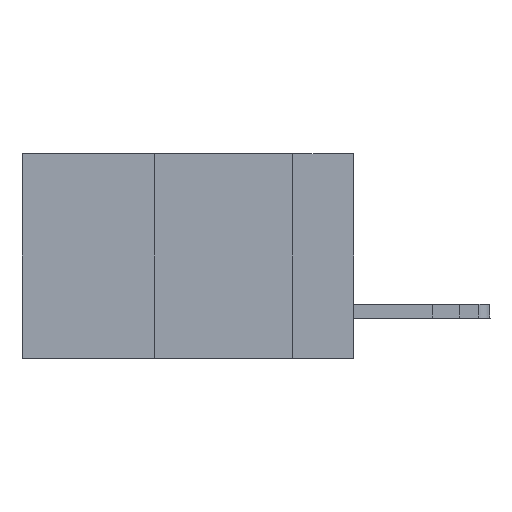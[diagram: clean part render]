
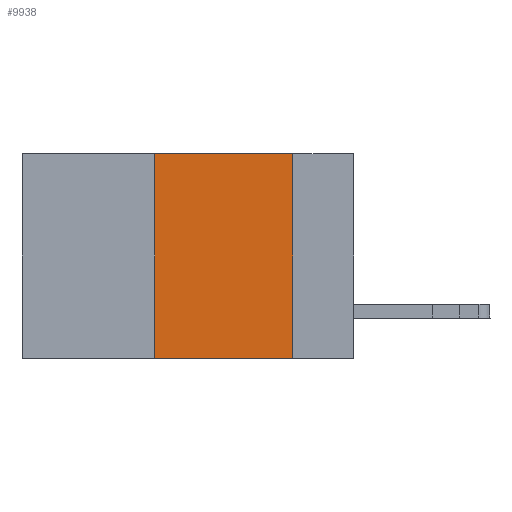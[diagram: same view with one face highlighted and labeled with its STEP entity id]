
A CAD part, left-side view. The second image highlights one B-rep face of the part: STEP entity #9938.
In plain terms, the highlighted planar face has unit normal (-1, 0, 0).
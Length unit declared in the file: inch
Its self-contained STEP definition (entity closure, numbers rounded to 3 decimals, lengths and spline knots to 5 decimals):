
#1124 = VERTEX_POINT ( 'NONE', #6725 ) ;
#1776 = LINE ( 'NONE', #12048, #10622 ) ;
#1821 = DIRECTION ( 'NONE',  ( 0., -1., 0. ) ) ;
#2107 = CARTESIAN_POINT ( 'NONE',  ( 0., 0.11, 0. ) ) ;
#3855 = CARTESIAN_POINT ( 'NONE',  ( 0., 0.11, 0. ) ) ;
#4981 = EDGE_CURVE ( 'NONE', #1124, #7231, #6101, .T. ) ;
#5998 = EDGE_CURVE ( 'NONE', #9878, #8299, #15876, .T. ) ;
#6101 = LINE ( 'NONE', #16797, #10992 ) ;
#6137 = CARTESIAN_POINT ( 'NONE',  ( 0., 0.36, 0. ) ) ;
#6437 = ORIENTED_EDGE ( 'NONE', *, *, #5998, .F. ) ;
#6725 = CARTESIAN_POINT ( 'NONE',  ( 0., 0.36, -0.37 ) ) ;
#7231 = VERTEX_POINT ( 'NONE', #14925 ) ;
#7925 = VECTOR ( 'NONE', #18541, 39.37008 ) ;
#8299 = VERTEX_POINT ( 'NONE', #3855 ) ;
#8394 = PLANE ( 'NONE',  #9184 ) ;
#8455 = DIRECTION ( 'NONE',  ( 0., 0., -1. ) ) ;
#9184 = AXIS2_PLACEMENT_3D ( 'NONE', #11413, #17451, #8455 ) ;
#9392 = ORIENTED_EDGE ( 'NONE', *, *, #9624, .F. ) ;
#9624 = EDGE_CURVE ( 'NONE', #1124, #9878, #1776, .T. ) ;
#9645 = CARTESIAN_POINT ( 'NONE',  ( 0., 0.6, 0. ) ) ;
#9878 = VERTEX_POINT ( 'NONE', #6137 ) ;
#9938 = ADVANCED_FACE ( 'NONE', ( #12784 ), #8394, .F. ) ;
#10622 = VECTOR ( 'NONE', #15670, 39.37008 ) ;
#10935 = EDGE_CURVE ( 'NONE', #8299, #7231, #18372, .T. ) ;
#10992 = VECTOR ( 'NONE', #1821, 39.37008 ) ;
#11109 = VECTOR ( 'NONE', #15543, 39.37008 ) ;
#11413 = CARTESIAN_POINT ( 'NONE',  ( 0., 0.6, 0. ) ) ;
#11495 = EDGE_LOOP ( 'NONE', ( #16876, #6437, #9392, #13695 ) ) ;
#12048 = CARTESIAN_POINT ( 'NONE',  ( 0., 0.36, 0. ) ) ;
#12784 = FACE_OUTER_BOUND ( 'NONE', #11495, .T. ) ;
#13695 = ORIENTED_EDGE ( 'NONE', *, *, #4981, .T. ) ;
#14925 = CARTESIAN_POINT ( 'NONE',  ( 0., 0.11, -0.37 ) ) ;
#15543 = DIRECTION ( 'NONE',  ( 0., 0., -1. ) ) ;
#15670 = DIRECTION ( 'NONE',  ( 0., 0., 1. ) ) ;
#15876 = LINE ( 'NONE', #9645, #7925 ) ;
#16797 = CARTESIAN_POINT ( 'NONE',  ( 0., 0.6, -0.37 ) ) ;
#16876 = ORIENTED_EDGE ( 'NONE', *, *, #10935, .F. ) ;
#17451 = DIRECTION ( 'NONE',  ( 1., 0., 0. ) ) ;
#18372 = LINE ( 'NONE', #2107, #11109 ) ;
#18541 = DIRECTION ( 'NONE',  ( 0., -1., 0. ) ) ;
